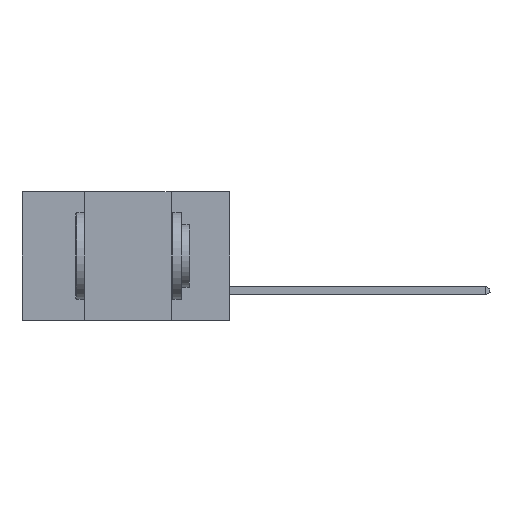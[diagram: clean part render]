
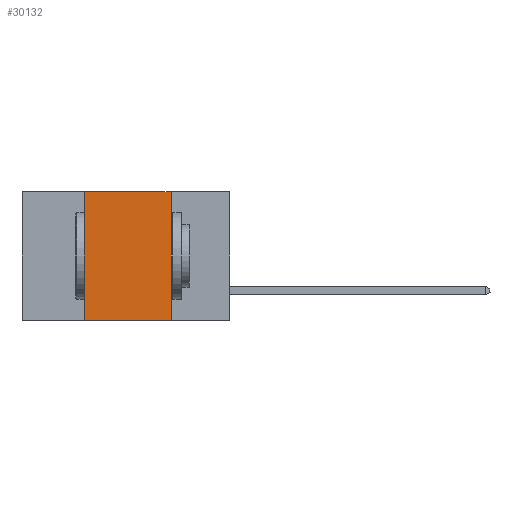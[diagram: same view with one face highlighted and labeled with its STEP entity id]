
A CAD part, left-side view. The second image highlights one B-rep face of the part: STEP entity #30132.
In plain terms, the highlighted planar face has unit normal (-1, 0, 0).
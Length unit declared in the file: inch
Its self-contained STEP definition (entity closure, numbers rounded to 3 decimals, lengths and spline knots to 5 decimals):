
#454 = VECTOR ( 'NONE', #27718, 39.37008 ) ;
#585 = EDGE_LOOP ( 'NONE', ( #26062, #11159, #15959, #1431 ) ) ;
#778 = DIRECTION ( 'NONE',  ( 0., -1., 0. ) ) ;
#1431 = ORIENTED_EDGE ( 'NONE', *, *, #4727, .T. ) ;
#1696 = DIRECTION ( 'NONE',  ( 0., 0., -1. ) ) ;
#1776 = CARTESIAN_POINT ( 'NONE',  ( 0., 0.6, 0. ) ) ;
#1797 = PLANE ( 'NONE',  #24063 ) ;
#3801 = DIRECTION ( 'NONE',  ( 0., 0., 1. ) ) ;
#4142 = DIRECTION ( 'NONE',  ( 1., 0., 0. ) ) ;
#4476 = LINE ( 'NONE', #1776, #454 ) ;
#4727 = EDGE_CURVE ( 'NONE', #27622, #6766, #16605, .T. ) ;
#6766 = VERTEX_POINT ( 'NONE', #9915 ) ;
#8654 = VECTOR ( 'NONE', #3801, 39.37008 ) ;
#9915 = CARTESIAN_POINT ( 'NONE',  ( 0., 0.17, -0.37 ) ) ;
#10853 = CARTESIAN_POINT ( 'NONE',  ( 0., 0.42, -0.37 ) ) ;
#11159 = ORIENTED_EDGE ( 'NONE', *, *, #12749, .F. ) ;
#12749 = EDGE_CURVE ( 'NONE', #22978, #24383, #4476, .T. ) ;
#13214 = CARTESIAN_POINT ( 'NONE',  ( 0., 0.17, 0. ) ) ;
#14739 = CARTESIAN_POINT ( 'NONE',  ( 0., 0.6, -0.37 ) ) ;
#14848 = LINE ( 'NONE', #27002, #8654 ) ;
#15435 = VECTOR ( 'NONE', #15641, 39.37008 ) ;
#15641 = DIRECTION ( 'NONE',  ( 0., 0., -1. ) ) ;
#15959 = ORIENTED_EDGE ( 'NONE', *, *, #27609, .F. ) ;
#16605 = LINE ( 'NONE', #14739, #30063 ) ;
#18725 = LINE ( 'NONE', #13214, #15435 ) ;
#21150 = CARTESIAN_POINT ( 'NONE',  ( 0., 0.42, 0. ) ) ;
#22931 = CARTESIAN_POINT ( 'NONE',  ( 0., 0.6, 0. ) ) ;
#22978 = VERTEX_POINT ( 'NONE', #21150 ) ;
#24063 = AXIS2_PLACEMENT_3D ( 'NONE', #22931, #4142, #1696 ) ;
#24383 = VERTEX_POINT ( 'NONE', #24946 ) ;
#24946 = CARTESIAN_POINT ( 'NONE',  ( 0., 0.17, 0. ) ) ;
#26062 = ORIENTED_EDGE ( 'NONE', *, *, #30038, .F. ) ;
#27002 = CARTESIAN_POINT ( 'NONE',  ( 0., 0.42, 0. ) ) ;
#27087 = FACE_OUTER_BOUND ( 'NONE', #585, .T. ) ;
#27609 = EDGE_CURVE ( 'NONE', #27622, #22978, #14848, .T. ) ;
#27622 = VERTEX_POINT ( 'NONE', #10853 ) ;
#27718 = DIRECTION ( 'NONE',  ( 0., -1., 0. ) ) ;
#30038 = EDGE_CURVE ( 'NONE', #24383, #6766, #18725, .T. ) ;
#30063 = VECTOR ( 'NONE', #778, 39.37008 ) ;
#30132 = ADVANCED_FACE ( 'NONE', ( #27087 ), #1797, .F. ) ;
